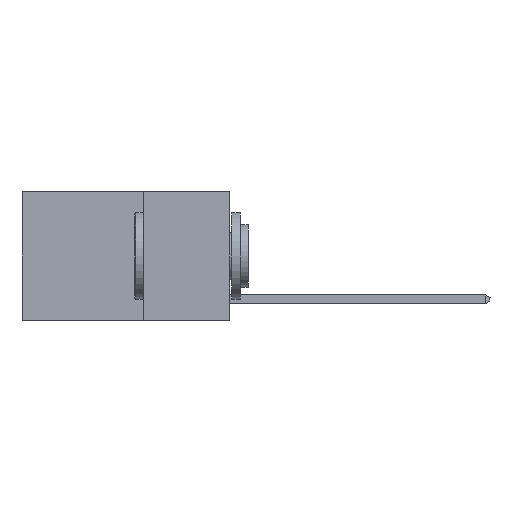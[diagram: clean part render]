
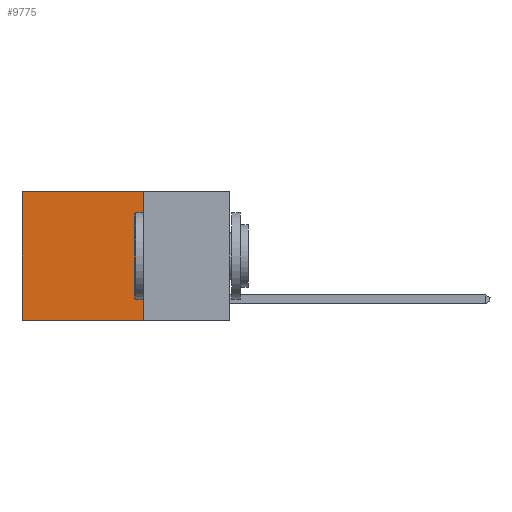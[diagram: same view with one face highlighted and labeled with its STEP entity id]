
A CAD part, left-side view. The second image highlights one B-rep face of the part: STEP entity #9775.
In plain terms, the highlighted planar face has unit normal (-1, 0, 0).
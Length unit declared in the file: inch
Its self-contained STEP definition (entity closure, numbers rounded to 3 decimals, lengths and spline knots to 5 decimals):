
#1526 = CARTESIAN_POINT ( 'NONE',  ( 0.2625, 0.25, 0. ) ) ;
#2356 = CARTESIAN_POINT ( 'NONE',  ( 0.2625, 0.6, -0.37 ) ) ;
#2611 = CARTESIAN_POINT ( 'NONE',  ( 0.2625, 0.25, 0. ) ) ;
#2642 = ORIENTED_EDGE ( 'NONE', *, *, #9655, .F. ) ;
#3489 = CARTESIAN_POINT ( 'NONE',  ( 0.2625, 0.6, 0. ) ) ;
#3821 = DIRECTION ( 'NONE',  ( 0., 1., 0. ) ) ;
#4354 = DIRECTION ( 'NONE',  ( 0., 0., -1. ) ) ;
#5591 = AXIS2_PLACEMENT_3D ( 'NONE', #2611, #22506, #4354 ) ;
#6686 = ORIENTED_EDGE ( 'NONE', *, *, #13932, .T. ) ;
#6720 = PLANE ( 'NONE',  #5591 ) ;
#7470 = EDGE_CURVE ( 'NONE', #14112, #14534, #8178, .T. ) ;
#7473 = LINE ( 'NONE', #23792, #23493 ) ;
#7656 = DIRECTION ( 'NONE',  ( 0., 1., 0. ) ) ;
#8178 = LINE ( 'NONE', #10026, #9739 ) ;
#8247 = ORIENTED_EDGE ( 'NONE', *, *, #14062, .F. ) ;
#8946 = LINE ( 'NONE', #25000, #10736 ) ;
#9655 = EDGE_CURVE ( 'NONE', #13521, #9791, #25829, .T. ) ;
#9739 = VECTOR ( 'NONE', #3821, 39.37008 ) ;
#9775 = ADVANCED_FACE ( 'NONE', ( #12281 ), #6720, .F. ) ;
#9791 = VERTEX_POINT ( 'NONE', #2356 ) ;
#10026 = CARTESIAN_POINT ( 'NONE',  ( 0.2625, 0.25, 0. ) ) ;
#10032 = CARTESIAN_POINT ( 'NONE',  ( 0.2625, 0.25, -0.37 ) ) ;
#10736 = VECTOR ( 'NONE', #22390, 39.37008 ) ;
#12281 = FACE_OUTER_BOUND ( 'NONE', #18923, .T. ) ;
#12463 = CARTESIAN_POINT ( 'NONE',  ( 0.2625, 0.25, -0.37 ) ) ;
#13198 = VECTOR ( 'NONE', #7656, 39.37008 ) ;
#13521 = VERTEX_POINT ( 'NONE', #12463 ) ;
#13932 = EDGE_CURVE ( 'NONE', #14534, #9791, #8946, .T. ) ;
#14062 = EDGE_CURVE ( 'NONE', #14112, #13521, #7473, .T. ) ;
#14112 = VERTEX_POINT ( 'NONE', #1526 ) ;
#14534 = VERTEX_POINT ( 'NONE', #3489 ) ;
#18923 = EDGE_LOOP ( 'NONE', ( #6686, #2642, #8247, #21451 ) ) ;
#21451 = ORIENTED_EDGE ( 'NONE', *, *, #7470, .T. ) ;
#22390 = DIRECTION ( 'NONE',  ( 0., 0., -1. ) ) ;
#22506 = DIRECTION ( 'NONE',  ( 1., 0., 0. ) ) ;
#23407 = DIRECTION ( 'NONE',  ( 0., 0., -1. ) ) ;
#23493 = VECTOR ( 'NONE', #23407, 39.37008 ) ;
#23792 = CARTESIAN_POINT ( 'NONE',  ( 0.2625, 0.25, 0. ) ) ;
#25000 = CARTESIAN_POINT ( 'NONE',  ( 0.2625, 0.6, 0. ) ) ;
#25829 = LINE ( 'NONE', #10032, #13198 ) ;
